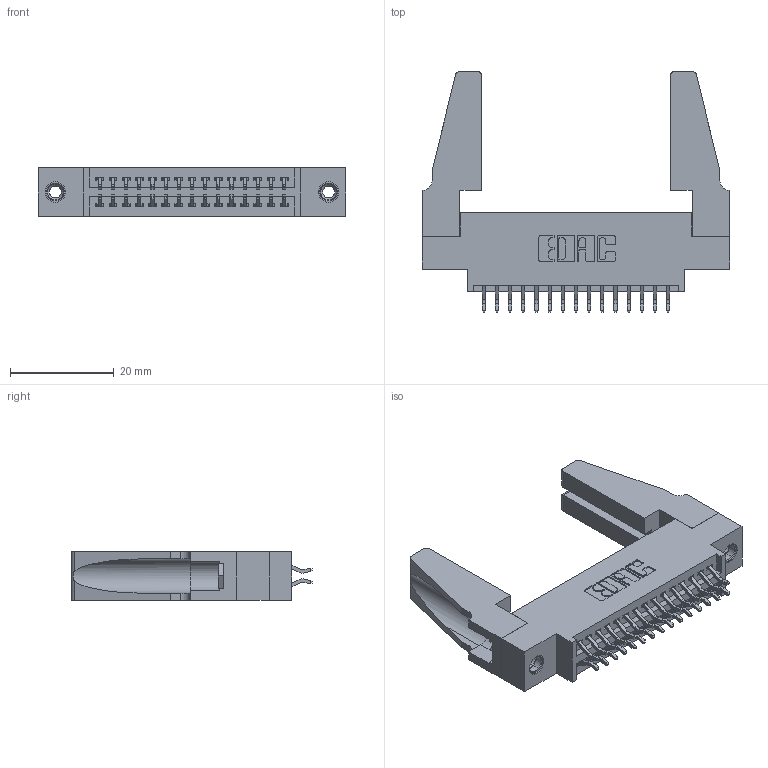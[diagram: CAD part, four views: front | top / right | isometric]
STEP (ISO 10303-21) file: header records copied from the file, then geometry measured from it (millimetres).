
FILE_DESCRIPTION (( 'STEP AP203' ), '1' );
FILE_NAME ('395-030-556-888.STEP', '2019-10-17T14:57:11', ( '' ), ( '' ), 'SwSTEP 2.0', 'SolidWorks 2016', '' );
FILE_SCHEMA (( 'CONFIG_CONTROL_DESIGN' ));
Length unit declared in the file: inch
Products named in the file (5): 345 Part_0.170 Offset - 0.156 Dia-TH; 345-292-001_556 Tail; 345-250-001_345-250-001-102; 345-220-078_345-220-088; 395-030-556-888
Assembly tree (35 placements, depth 2):
  395-030-556-888
    345 Part_0.170 Offset - 0.156 Dia-TH
    345-292-001_556 Tail  x30
    345-250-001_345-250-001-102  x2
    345-220-078_345-220-088  x2
Bounding box: 59.33 x 46.41 x 9.4 mm (x, y, z)
Volume: 8651.1 mm3; surface area: 10696.5 mm2
Topology: 35 solids, 35 shells, 1934 faces, 5677 edges, 3734 vertices
Faces by surface type: plane 1266, cylinder 652, cone 12, torus 4
Entity records: 17904 total; most frequent: CARTESIAN_POINT 3038, ORIENTED_EDGE 2920, DIRECTION 2704, EDGE_CURVE 1460, VECTOR 1218, LINE 1218, VERTEX_POINT 966, AXIS2_PLACEMENT_3D 743
